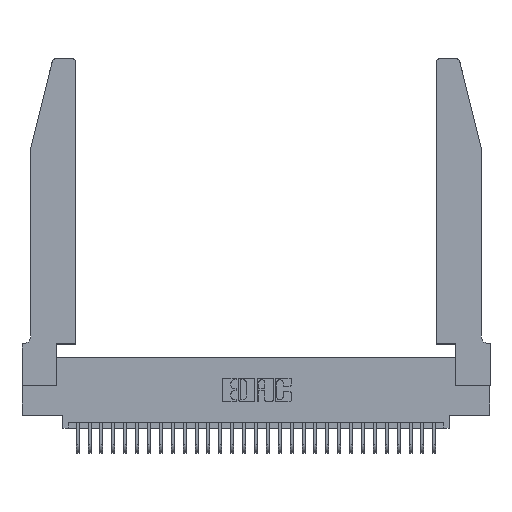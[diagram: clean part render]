
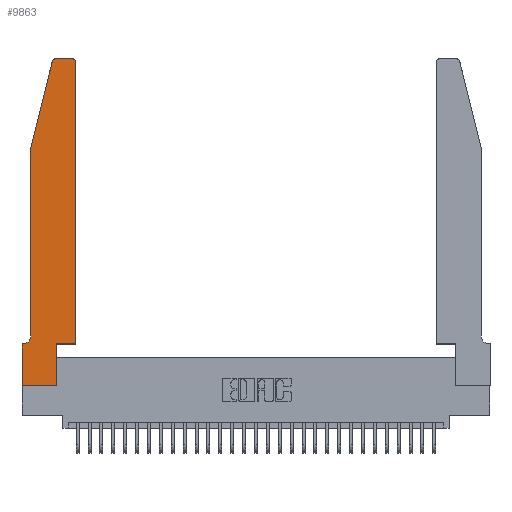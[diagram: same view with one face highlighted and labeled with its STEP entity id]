
A CAD part, top view. The second image highlights one B-rep face of the part: STEP entity #9863.
In plain terms, the highlighted planar face has unit normal (0, 0, 1).
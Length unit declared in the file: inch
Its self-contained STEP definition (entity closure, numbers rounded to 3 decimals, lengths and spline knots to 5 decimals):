
#156 = CARTESIAN_POINT ( 'NONE',  ( 0.2865, 0.35, 0.37 ) ) ;
#247 = VERTEX_POINT ( 'NONE', #29774 ) ;
#312 = LINE ( 'NONE', #14263, #31968 ) ;
#930 = EDGE_CURVE ( 'NONE', #18503, #247, #312, .T. ) ;
#1134 = ORIENTED_EDGE ( 'NONE', *, *, #8466, .T. ) ;
#1267 = EDGE_CURVE ( 'NONE', #31643, #18503, #18846, .T. ) ;
#1543 = CARTESIAN_POINT ( 'NONE',  ( 0.2865, 0.35, 0.37 ) ) ;
#1734 = ORIENTED_EDGE ( 'NONE', *, *, #6921, .T. ) ;
#1917 = LINE ( 'NONE', #7053, #7982 ) ;
#2240 = CARTESIAN_POINT ( 'NONE',  ( 0.2605, 2.75, 0.37 ) ) ;
#2472 = DIRECTION ( 'NONE',  ( -1., 0., 0. ) ) ;
#2824 = LINE ( 'NONE', #14965, #15450 ) ;
#3372 = VECTOR ( 'NONE', #2472, 39.37008 ) ;
#3480 = VERTEX_POINT ( 'NONE', #19459 ) ;
#4741 = CARTESIAN_POINT ( 'NONE',  ( 0.284, 2.72, 0.37 ) ) ;
#4768 = CARTESIAN_POINT ( 'NONE',  ( 0.0755, 0.42, 0.37 ) ) ;
#5099 = CARTESIAN_POINT ( 'NONE',  ( 0.284, 2.75, 0.37 ) ) ;
#5184 = VECTOR ( 'NONE', #13210, 39.37008 ) ;
#5479 = DIRECTION ( 'NONE',  ( 0., -1., 0. ) ) ;
#6129 = EDGE_CURVE ( 'NONE', #25101, #3480, #19268, .T. ) ;
#6591 = CARTESIAN_POINT ( 'NONE',  ( 0.0755, 2., 0.37 ) ) ;
#6612 = CARTESIAN_POINT ( 'NONE',  ( 0.25487, 2.72718, 0.37 ) ) ;
#6886 = CARTESIAN_POINT ( 'NONE',  ( 0., 0.35, 0.37 ) ) ;
#6921 = EDGE_CURVE ( 'NONE', #9401, #25508, #10713, .T. ) ;
#7053 = CARTESIAN_POINT ( 'NONE',  ( 0.0755, 2., 0.37 ) ) ;
#7199 = VERTEX_POINT ( 'NONE', #8287 ) ;
#7338 = DIRECTION ( 'NONE',  ( 1., 0., 0. ) ) ;
#7530 = CARTESIAN_POINT ( 'NONE',  ( 0.4505, 2.72, 0.37 ) ) ;
#7982 = VECTOR ( 'NONE', #23759, 39.37008 ) ;
#8287 = CARTESIAN_POINT ( 'NONE',  ( 0.2865, 0., 0.37 ) ) ;
#8374 = VERTEX_POINT ( 'NONE', #30969 ) ;
#8466 = EDGE_CURVE ( 'NONE', #8374, #25101, #32195, .T. ) ;
#8828 = EDGE_CURVE ( 'NONE', #247, #13421, #30283, .T. ) ;
#8913 = DIRECTION ( 'NONE',  ( 0., 0., 1. ) ) ;
#9099 = DIRECTION ( 'NONE',  ( -0.239, -0.971, 0. ) ) ;
#9389 = DIRECTION ( 'NONE',  ( 1., 0., 0. ) ) ;
#9401 = VERTEX_POINT ( 'NONE', #5099 ) ;
#9803 = VECTOR ( 'NONE', #5479, 39.37008 ) ;
#9863 = ADVANCED_FACE ( 'NONE', ( #14197 ), #21717, .T. ) ;
#9933 = AXIS2_PLACEMENT_3D ( 'NONE', #23671, #8913, #26178 ) ;
#10201 = EDGE_CURVE ( 'NONE', #26160, #8374, #24169, .T. ) ;
#10713 = CIRCLE ( 'NONE', #20306, 0.03 ) ;
#10942 = VECTOR ( 'NONE', #9099, 39.37008 ) ;
#11256 = ORIENTED_EDGE ( 'NONE', *, *, #15697, .T. ) ;
#11797 = CARTESIAN_POINT ( 'NONE',  ( 0.0055, 0.35, 0.37 ) ) ;
#12281 = ORIENTED_EDGE ( 'NONE', *, *, #10201, .T. ) ;
#12986 = EDGE_CURVE ( 'NONE', #3480, #9401, #16738, .T. ) ;
#13210 = DIRECTION ( 'NONE',  ( 1., 0., 0. ) ) ;
#13421 = VERTEX_POINT ( 'NONE', #24239 ) ;
#14059 = ORIENTED_EDGE ( 'NONE', *, *, #24717, .T. ) ;
#14197 = FACE_OUTER_BOUND ( 'NONE', #29006, .T. ) ;
#14263 = CARTESIAN_POINT ( 'NONE',  ( 0.0755, 0.35, 0.37 ) ) ;
#14586 = ORIENTED_EDGE ( 'NONE', *, *, #22678, .T. ) ;
#14819 = LINE ( 'NONE', #6591, #10942 ) ;
#14965 = CARTESIAN_POINT ( 'NONE',  ( 0., 0., 0.37 ) ) ;
#15037 = CARTESIAN_POINT ( 'NONE',  ( 0.0755, 2., 0.37 ) ) ;
#15450 = VECTOR ( 'NONE', #24803, 39.37008 ) ;
#15697 = EDGE_CURVE ( 'NONE', #7199, #26160, #21191, .T. ) ;
#16060 = ORIENTED_EDGE ( 'NONE', *, *, #8828, .T. ) ;
#16738 = LINE ( 'NONE', #2240, #3372 ) ;
#16916 = ORIENTED_EDGE ( 'NONE', *, *, #1267, .T. ) ;
#18503 = VERTEX_POINT ( 'NONE', #11797 ) ;
#18706 = VERTEX_POINT ( 'NONE', #15037 ) ;
#18846 = CIRCLE ( 'NONE', #23464, 0.07 ) ;
#19268 = CIRCLE ( 'NONE', #9933, 0.03 ) ;
#19459 = CARTESIAN_POINT ( 'NONE',  ( 0.4205, 2.75, 0.37 ) ) ;
#20306 = AXIS2_PLACEMENT_3D ( 'NONE', #4741, #22155, #7338 ) ;
#20336 = DIRECTION ( 'NONE',  ( 0., 1., 0. ) ) ;
#20387 = CARTESIAN_POINT ( 'NONE',  ( 0., 0., 0.37 ) ) ;
#20625 = DIRECTION ( 'NONE',  ( -1., 0., 0. ) ) ;
#21191 = LINE ( 'NONE', #156, #26961 ) ;
#21717 = PLANE ( 'NONE',  #23143 ) ;
#22155 = DIRECTION ( 'NONE',  ( 0., 0., 1. ) ) ;
#22678 = EDGE_CURVE ( 'NONE', #25508, #18706, #14819, .T. ) ;
#22861 = ORIENTED_EDGE ( 'NONE', *, *, #930, .T. ) ;
#23143 = AXIS2_PLACEMENT_3D ( 'NONE', #6886, #24127, #9389 ) ;
#23464 = AXIS2_PLACEMENT_3D ( 'NONE', #24461, #29185, #29288 ) ;
#23671 = CARTESIAN_POINT ( 'NONE',  ( 0.4205, 2.72, 0.37 ) ) ;
#23759 = DIRECTION ( 'NONE',  ( 0., -1., 0. ) ) ;
#23902 = CARTESIAN_POINT ( 'NONE',  ( 0.4505, 0.35, 0.37 ) ) ;
#24127 = DIRECTION ( 'NONE',  ( 0., 0., 1. ) ) ;
#24169 = LINE ( 'NONE', #25428, #5184 ) ;
#24239 = CARTESIAN_POINT ( 'NONE',  ( 0., 0., 0.37 ) ) ;
#24461 = CARTESIAN_POINT ( 'NONE',  ( 0.0055, 0.42, 0.37 ) ) ;
#24662 = ORIENTED_EDGE ( 'NONE', *, *, #30198, .T. ) ;
#24717 = EDGE_CURVE ( 'NONE', #13421, #7199, #2824, .T. ) ;
#24803 = DIRECTION ( 'NONE',  ( 1., 0., 0. ) ) ;
#24821 = VECTOR ( 'NONE', #31392, 39.37008 ) ;
#25101 = VERTEX_POINT ( 'NONE', #7530 ) ;
#25341 = ORIENTED_EDGE ( 'NONE', *, *, #6129, .T. ) ;
#25428 = CARTESIAN_POINT ( 'NONE',  ( 0.4505, 0.35, 0.37 ) ) ;
#25508 = VERTEX_POINT ( 'NONE', #6612 ) ;
#26160 = VERTEX_POINT ( 'NONE', #1543 ) ;
#26178 = DIRECTION ( 'NONE',  ( 1., 0., 0. ) ) ;
#26961 = VECTOR ( 'NONE', #20336, 39.37008 ) ;
#29006 = EDGE_LOOP ( 'NONE', ( #31385, #1734, #14586, #24662, #16916, #22861, #16060, #14059, #11256, #12281, #1134, #25341 ) ) ;
#29185 = DIRECTION ( 'NONE',  ( 0., 0., -1. ) ) ;
#29288 = DIRECTION ( 'NONE',  ( -1., 0., 0. ) ) ;
#29774 = CARTESIAN_POINT ( 'NONE',  ( 0., 0.35, 0.37 ) ) ;
#30198 = EDGE_CURVE ( 'NONE', #18706, #31643, #1917, .T. ) ;
#30283 = LINE ( 'NONE', #20387, #9803 ) ;
#30969 = CARTESIAN_POINT ( 'NONE',  ( 0.4505, 0.35, 0.37 ) ) ;
#31385 = ORIENTED_EDGE ( 'NONE', *, *, #12986, .T. ) ;
#31392 = DIRECTION ( 'NONE',  ( 0., 1., 0. ) ) ;
#31643 = VERTEX_POINT ( 'NONE', #4768 ) ;
#31968 = VECTOR ( 'NONE', #20625, 39.37008 ) ;
#32195 = LINE ( 'NONE', #23902, #24821 ) ;
